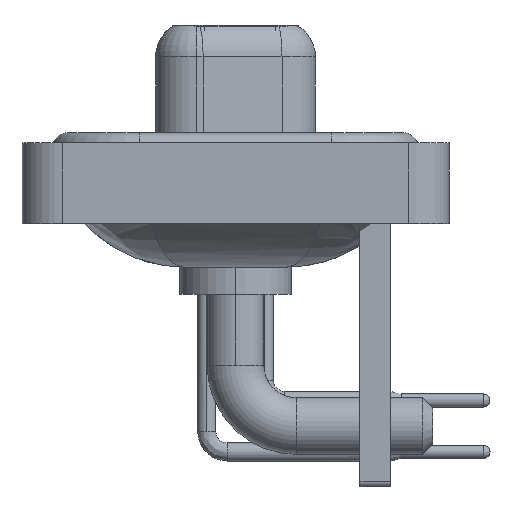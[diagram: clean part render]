
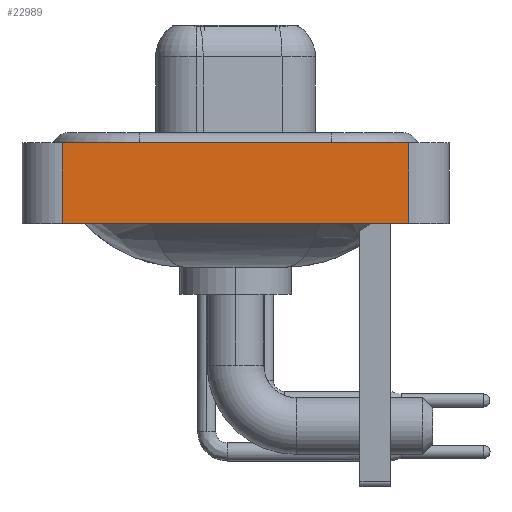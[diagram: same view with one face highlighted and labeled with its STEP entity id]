
A CAD part, left-side view. The second image highlights one B-rep face of the part: STEP entity #22989.
In plain terms, the highlighted planar face has unit normal (-1, 0, 0).
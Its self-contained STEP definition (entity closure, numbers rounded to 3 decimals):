
#108 = CARTESIAN_POINT ( 'NONE',  ( -7.35, -8.55, -3.6 ) ) ;
#277 = CARTESIAN_POINT ( 'NONE',  ( -7.35, 8.55, -3.6 ) ) ;
#528 = VERTEX_POINT ( 'NONE', #24599 ) ;
#1710 = CARTESIAN_POINT ( 'NONE',  ( -7.35, -8.55, -3.6 ) ) ;
#2381 = CARTESIAN_POINT ( 'NONE',  ( -7.35, -8.55, -3.6 ) ) ;
#4166 = VECTOR ( 'NONE', #10418, 1000. ) ;
#5084 = EDGE_CURVE ( 'NONE', #6760, #21885, #21013, .T. ) ;
#5744 = EDGE_CURVE ( 'NONE', #5864, #528, #22105, .T. ) ;
#5864 = VERTEX_POINT ( 'NONE', #20673 ) ;
#6084 = DIRECTION ( 'NONE',  ( 0., 0., 1. ) ) ;
#6760 = VERTEX_POINT ( 'NONE', #9513 ) ;
#6791 = DIRECTION ( 'NONE',  ( 0., -1., 0. ) ) ;
#8734 = AXIS2_PLACEMENT_3D ( 'NONE', #21812, #19378, #15993 ) ;
#9513 = CARTESIAN_POINT ( 'NONE',  ( -7.35, 8.55, -3.6 ) ) ;
#9678 = VECTOR ( 'NONE', #6791, 1000. ) ;
#9986 = PLANE ( 'NONE',  #8734 ) ;
#10418 = DIRECTION ( 'NONE',  ( 0., 0., 1. ) ) ;
#11489 = LINE ( 'NONE', #277, #15290 ) ;
#14073 = ORIENTED_EDGE ( 'NONE', *, *, #5084, .T. ) ;
#14355 = CARTESIAN_POINT ( 'NONE',  ( -7.35, -8.55, 0.4 ) ) ;
#15290 = VECTOR ( 'NONE', #6084, 1000. ) ;
#15750 = ORIENTED_EDGE ( 'NONE', *, *, #20809, .T. ) ;
#15993 = DIRECTION ( 'NONE',  ( 0., 0., 1. ) ) ;
#17890 = LINE ( 'NONE', #108, #4166 ) ;
#19214 = DIRECTION ( 'NONE',  ( 0., -1., 0. ) ) ;
#19378 = DIRECTION ( 'NONE',  ( -1., 0., 0. ) ) ;
#19506 = FACE_OUTER_BOUND ( 'NONE', #22899, .T. ) ;
#19941 = VECTOR ( 'NONE', #19214, 1000. ) ;
#20673 = CARTESIAN_POINT ( 'NONE',  ( -7.35, 8.55, 0.4 ) ) ;
#20809 = EDGE_CURVE ( 'NONE', #21885, #528, #17890, .T. ) ;
#21013 = LINE ( 'NONE', #1710, #19941 ) ;
#21756 = ORIENTED_EDGE ( 'NONE', *, *, #24673, .F. ) ;
#21812 = CARTESIAN_POINT ( 'NONE',  ( -7.35, -8.55, -3.6 ) ) ;
#21885 = VERTEX_POINT ( 'NONE', #2381 ) ;
#22105 = LINE ( 'NONE', #14355, #9678 ) ;
#22899 = EDGE_LOOP ( 'NONE', ( #15750, #22996, #21756, #14073 ) ) ;
#22989 = ADVANCED_FACE ( 'NONE', ( #19506 ), #9986, .T. ) ;
#22996 = ORIENTED_EDGE ( 'NONE', *, *, #5744, .F. ) ;
#24599 = CARTESIAN_POINT ( 'NONE',  ( -7.35, -8.55, 0.4 ) ) ;
#24673 = EDGE_CURVE ( 'NONE', #6760, #5864, #11489, .T. ) ;
